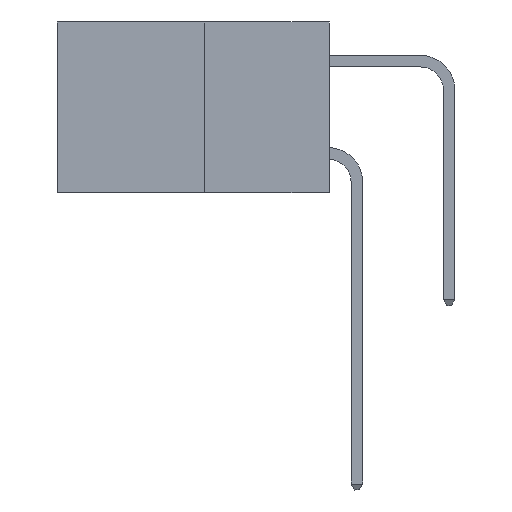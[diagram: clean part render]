
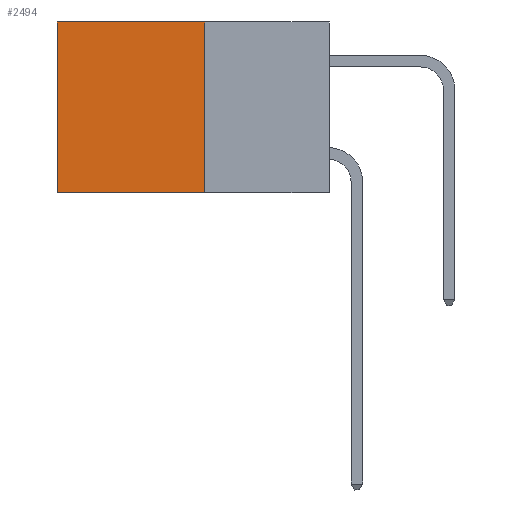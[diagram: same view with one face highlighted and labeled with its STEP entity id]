
A CAD part, left-side view. The second image highlights one B-rep face of the part: STEP entity #2494.
In plain terms, the highlighted planar face has unit normal (-1, 0, 0).
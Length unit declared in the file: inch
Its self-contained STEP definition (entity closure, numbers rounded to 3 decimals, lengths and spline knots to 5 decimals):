
#315 = DIRECTION ( 'NONE',  ( 0., 1., 0. ) ) ;
#706 = ORIENTED_EDGE ( 'NONE', *, *, #10893, .F. ) ;
#759 = ORIENTED_EDGE ( 'NONE', *, *, #6791, .T. ) ;
#841 = LINE ( 'NONE', #10092, #3252 ) ;
#961 = AXIS2_PLACEMENT_3D ( 'NONE', #5158, #2717, #1865 ) ;
#1865 = DIRECTION ( 'NONE',  ( 0., 0., -1. ) ) ;
#2050 = CARTESIAN_POINT ( 'NONE',  ( 0.277, 0.59, 0. ) ) ;
#2494 = ADVANCED_FACE ( 'NONE', ( #3287 ), #6955, .F. ) ;
#2668 = DIRECTION ( 'NONE',  ( 0., 0., -1. ) ) ;
#2704 = VECTOR ( 'NONE', #2668, 39.37008 ) ;
#2717 = DIRECTION ( 'NONE',  ( 1., 0., 0. ) ) ;
#3094 = CARTESIAN_POINT ( 'NONE',  ( 0.277, 0.27, -0.37 ) ) ;
#3252 = VECTOR ( 'NONE', #10132, 39.37008 ) ;
#3287 = FACE_OUTER_BOUND ( 'NONE', #4004, .T. ) ;
#3494 = EDGE_CURVE ( 'NONE', #4339, #9221, #6484, .T. ) ;
#3816 = EDGE_CURVE ( 'NONE', #4339, #6514, #841, .T. ) ;
#3952 = CARTESIAN_POINT ( 'NONE',  ( 0.277, 0.27, 0. ) ) ;
#4004 = EDGE_LOOP ( 'NONE', ( #759, #706, #6980, #4255 ) ) ;
#4255 = ORIENTED_EDGE ( 'NONE', *, *, #3494, .T. ) ;
#4339 = VERTEX_POINT ( 'NONE', #3952 ) ;
#5158 = CARTESIAN_POINT ( 'NONE',  ( 0.277, 0.27, -0.37 ) ) ;
#6484 = LINE ( 'NONE', #9173, #8454 ) ;
#6514 = VERTEX_POINT ( 'NONE', #6612 ) ;
#6612 = CARTESIAN_POINT ( 'NONE',  ( 0.277, 0.27, -0.37 ) ) ;
#6661 = VERTEX_POINT ( 'NONE', #10123 ) ;
#6791 = EDGE_CURVE ( 'NONE', #9221, #6661, #9527, .T. ) ;
#6940 = CARTESIAN_POINT ( 'NONE',  ( 0.277, 0.59, -0.37 ) ) ;
#6955 = PLANE ( 'NONE',  #961 ) ;
#6980 = ORIENTED_EDGE ( 'NONE', *, *, #3816, .F. ) ;
#7528 = VECTOR ( 'NONE', #8168, 39.37008 ) ;
#7781 = LINE ( 'NONE', #3094, #7528 ) ;
#8168 = DIRECTION ( 'NONE',  ( 0., 1., 0. ) ) ;
#8454 = VECTOR ( 'NONE', #315, 39.37008 ) ;
#9173 = CARTESIAN_POINT ( 'NONE',  ( 0.277, 0.27, 0. ) ) ;
#9221 = VERTEX_POINT ( 'NONE', #2050 ) ;
#9527 = LINE ( 'NONE', #6940, #2704 ) ;
#10092 = CARTESIAN_POINT ( 'NONE',  ( 0.277, 0.27, -0.37 ) ) ;
#10123 = CARTESIAN_POINT ( 'NONE',  ( 0.277, 0.59, -0.37 ) ) ;
#10132 = DIRECTION ( 'NONE',  ( 0., 0., -1. ) ) ;
#10893 = EDGE_CURVE ( 'NONE', #6514, #6661, #7781, .T. ) ;
